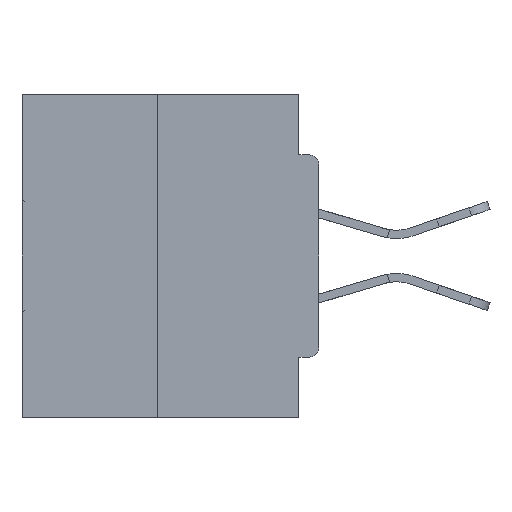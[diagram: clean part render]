
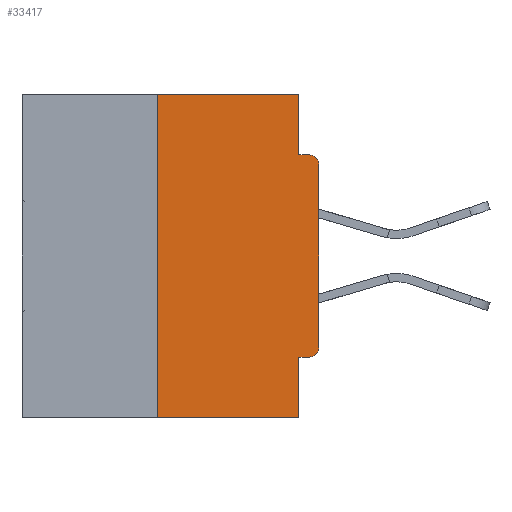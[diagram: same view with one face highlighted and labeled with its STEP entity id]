
A CAD part, left-side view. The second image highlights one B-rep face of the part: STEP entity #33417.
In plain terms, the highlighted planar face has unit normal (-1, 0, 0).
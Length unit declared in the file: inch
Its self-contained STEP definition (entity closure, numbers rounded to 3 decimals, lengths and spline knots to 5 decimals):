
#133 = CARTESIAN_POINT ( 'NONE',  ( 0., 0.46, -0.5 ) ) ;
#451 = CARTESIAN_POINT ( 'NONE',  ( 0., 0.46, 0. ) ) ;
#1035 = DIRECTION ( 'NONE',  ( 0., 0., 1. ) ) ;
#1209 = ORIENTED_EDGE ( 'NONE', *, *, #11673, .T. ) ;
#1415 = VECTOR ( 'NONE', #1035, 39.37008 ) ;
#1464 = CARTESIAN_POINT ( 'NONE',  ( 0., 0., -0.3915 ) ) ;
#2508 = DIRECTION ( 'NONE',  ( 0., 0., -1. ) ) ;
#2602 = CARTESIAN_POINT ( 'NONE',  ( 0., 0.031, -0.5 ) ) ;
#3315 = DIRECTION ( 'NONE',  ( 0., -1., 0. ) ) ;
#4146 = AXIS2_PLACEMENT_3D ( 'NONE', #15226, #35108, #2508 ) ;
#4529 = VERTEX_POINT ( 'NONE', #22738 ) ;
#5520 = LINE ( 'NONE', #41785, #1415 ) ;
#5610 = VECTOR ( 'NONE', #32253, 39.37008 ) ;
#5697 = VECTOR ( 'NONE', #22107, 39.37008 ) ;
#6129 = CARTESIAN_POINT ( 'NONE',  ( 0., 0.031, -0.0935 ) ) ;
#6334 = FACE_OUTER_BOUND ( 'NONE', #41774, .T. ) ;
#6608 = CARTESIAN_POINT ( 'NONE',  ( 0., 0., -0.1085 ) ) ;
#6823 = CARTESIAN_POINT ( 'NONE',  ( 0., 0.015, -0.4065 ) ) ;
#7087 = EDGE_CURVE ( 'NONE', #28979, #13288, #22943, .T. ) ;
#7140 = VECTOR ( 'NONE', #22441, 39.37008 ) ;
#7515 = VERTEX_POINT ( 'NONE', #9911 ) ;
#9369 = CARTESIAN_POINT ( 'NONE',  ( 0., 0., -0.4065 ) ) ;
#9911 = CARTESIAN_POINT ( 'NONE',  ( 0., 0.031, 0. ) ) ;
#10057 = ORIENTED_EDGE ( 'NONE', *, *, #33665, .F. ) ;
#10305 = AXIS2_PLACEMENT_3D ( 'NONE', #16853, #34337, #30231 ) ;
#11673 = EDGE_CURVE ( 'NONE', #34170, #20590, #32965, .T. ) ;
#12746 = CARTESIAN_POINT ( 'NONE',  ( 0., 0.031, -0.5 ) ) ;
#12936 = VERTEX_POINT ( 'NONE', #6823 ) ;
#13288 = VERTEX_POINT ( 'NONE', #22315 ) ;
#13840 = EDGE_CURVE ( 'NONE', #12936, #36607, #35130, .T. ) ;
#15226 = CARTESIAN_POINT ( 'NONE',  ( 0., 0.015, -0.1085 ) ) ;
#15431 = CARTESIAN_POINT ( 'NONE',  ( 0., 0.031, 0. ) ) ;
#16446 = DIRECTION ( 'NONE',  ( 0., 0., -1. ) ) ;
#16853 = CARTESIAN_POINT ( 'NONE',  ( 0., 0.015, -0.3915 ) ) ;
#17758 = EDGE_CURVE ( 'NONE', #19800, #13288, #33129, .T. ) ;
#19316 = VECTOR ( 'NONE', #36135, 39.37008 ) ;
#19334 = VERTEX_POINT ( 'NONE', #32987 ) ;
#19800 = VERTEX_POINT ( 'NONE', #6608 ) ;
#20042 = EDGE_CURVE ( 'NONE', #12936, #19334, #28139, .T. ) ;
#20201 = EDGE_CURVE ( 'NONE', #36607, #19800, #29635, .T. ) ;
#20590 = VERTEX_POINT ( 'NONE', #12746 ) ;
#21326 = ORIENTED_EDGE ( 'NONE', *, *, #7087, .F. ) ;
#22107 = DIRECTION ( 'NONE',  ( 0., 0., -1. ) ) ;
#22315 = CARTESIAN_POINT ( 'NONE',  ( 0., 0.015, -0.0935 ) ) ;
#22441 = DIRECTION ( 'NONE',  ( 0., 0., -1. ) ) ;
#22486 = ORIENTED_EDGE ( 'NONE', *, *, #13840, .T. ) ;
#22738 = CARTESIAN_POINT ( 'NONE',  ( 0., 0.25, 0. ) ) ;
#22756 = EDGE_CURVE ( 'NONE', #4529, #7515, #25964, .T. ) ;
#22928 = DIRECTION ( 'NONE',  ( 1., 0., 0. ) ) ;
#22943 = LINE ( 'NONE', #32467, #19316 ) ;
#23520 = ORIENTED_EDGE ( 'NONE', *, *, #22756, .F. ) ;
#24336 = AXIS2_PLACEMENT_3D ( 'NONE', #451, #22928, #16446 ) ;
#24821 = ORIENTED_EDGE ( 'NONE', *, *, #20201, .T. ) ;
#24848 = VECTOR ( 'NONE', #32684, 39.37008 ) ;
#25458 = LINE ( 'NONE', #2602, #7140 ) ;
#25964 = LINE ( 'NONE', #39373, #41639 ) ;
#26448 = ORIENTED_EDGE ( 'NONE', *, *, #35250, .F. ) ;
#26544 = ORIENTED_EDGE ( 'NONE', *, *, #39428, .F. ) ;
#26693 = CARTESIAN_POINT ( 'NONE',  ( 0., 0.25, -0.5 ) ) ;
#27390 = VECTOR ( 'NONE', #29935, 39.37008 ) ;
#28112 = ORIENTED_EDGE ( 'NONE', *, *, #17758, .T. ) ;
#28139 = LINE ( 'NONE', #9369, #5610 ) ;
#28979 = VERTEX_POINT ( 'NONE', #6129 ) ;
#29635 = LINE ( 'NONE', #29857, #24848 ) ;
#29857 = CARTESIAN_POINT ( 'NONE',  ( 0., 0., 0. ) ) ;
#29935 = DIRECTION ( 'NONE',  ( 0., -1., 0. ) ) ;
#30044 = PLANE ( 'NONE',  #24336 ) ;
#30231 = DIRECTION ( 'NONE',  ( 0., 0., -1. ) ) ;
#31853 = LINE ( 'NONE', #15431, #5697 ) ;
#32253 = DIRECTION ( 'NONE',  ( 0., 1., 0. ) ) ;
#32467 = CARTESIAN_POINT ( 'NONE',  ( 0., 0., -0.0935 ) ) ;
#32684 = DIRECTION ( 'NONE',  ( 0., 0., 1. ) ) ;
#32965 = LINE ( 'NONE', #133, #27390 ) ;
#32987 = CARTESIAN_POINT ( 'NONE',  ( 0., 0.031, -0.4065 ) ) ;
#33129 = CIRCLE ( 'NONE', #4146, 0.015 ) ;
#33417 = ADVANCED_FACE ( 'NONE', ( #6334 ), #30044, .F. ) ;
#33665 = EDGE_CURVE ( 'NONE', #19334, #20590, #25458, .T. ) ;
#34170 = VERTEX_POINT ( 'NONE', #26693 ) ;
#34337 = DIRECTION ( 'NONE',  ( -1., 0., 0. ) ) ;
#35108 = DIRECTION ( 'NONE',  ( -1., 0., 0. ) ) ;
#35130 = CIRCLE ( 'NONE', #10305, 0.015 ) ;
#35250 = EDGE_CURVE ( 'NONE', #34170, #4529, #5520, .T. ) ;
#36135 = DIRECTION ( 'NONE',  ( 0., -1., 0. ) ) ;
#36607 = VERTEX_POINT ( 'NONE', #1464 ) ;
#39373 = CARTESIAN_POINT ( 'NONE',  ( 0., 0.46, 0. ) ) ;
#39428 = EDGE_CURVE ( 'NONE', #7515, #28979, #31853, .T. ) ;
#41188 = ORIENTED_EDGE ( 'NONE', *, *, #20042, .F. ) ;
#41639 = VECTOR ( 'NONE', #3315, 39.37008 ) ;
#41774 = EDGE_LOOP ( 'NONE', ( #23520, #26448, #1209, #10057, #41188, #22486, #24821, #28112, #21326, #26544 ) ) ;
#41785 = CARTESIAN_POINT ( 'NONE',  ( 0., 0.25, 0. ) ) ;
